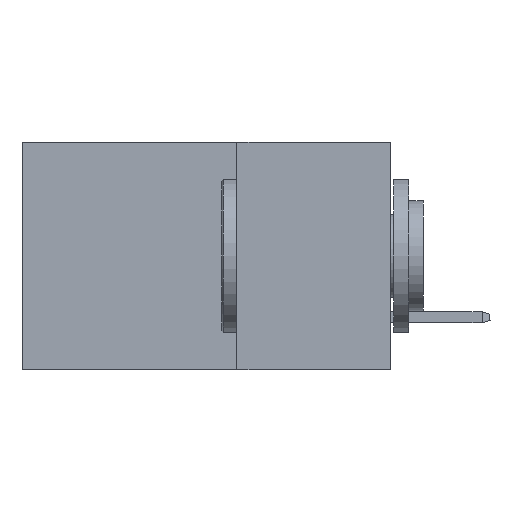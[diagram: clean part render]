
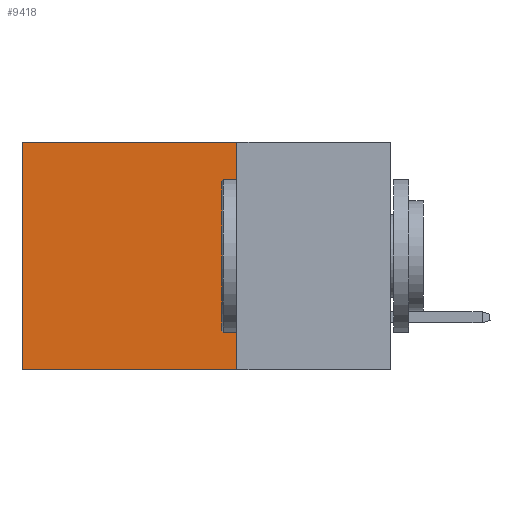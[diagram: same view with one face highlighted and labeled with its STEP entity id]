
A CAD part, left-side view. The second image highlights one B-rep face of the part: STEP entity #9418.
In plain terms, the highlighted planar face has unit normal (-1, 0, 0).
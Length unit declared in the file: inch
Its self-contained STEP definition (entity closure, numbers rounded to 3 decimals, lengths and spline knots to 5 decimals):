
#917 = VERTEX_POINT ( 'NONE', #14711 ) ;
#943 = LINE ( 'NONE', #15802, #15309 ) ;
#1311 = CARTESIAN_POINT ( 'NONE',  ( 0.2875, 0.6, -0.37 ) ) ;
#1991 = EDGE_CURVE ( 'NONE', #12289, #7194, #943, .T. ) ;
#3785 = CARTESIAN_POINT ( 'NONE',  ( 0.2875, 0.25, 0. ) ) ;
#4096 = ORIENTED_EDGE ( 'NONE', *, *, #1991, .T. ) ;
#4199 = LINE ( 'NONE', #7484, #7371 ) ;
#4247 = CARTESIAN_POINT ( 'NONE',  ( 0.2875, 0.25, 0. ) ) ;
#4553 = EDGE_CURVE ( 'NONE', #917, #7194, #4199, .T. ) ;
#4622 = CARTESIAN_POINT ( 'NONE',  ( 0.2875, 0.6, 0. ) ) ;
#6776 = FACE_OUTER_BOUND ( 'NONE', #11132, .T. ) ;
#7194 = VERTEX_POINT ( 'NONE', #1311 ) ;
#7371 = VECTOR ( 'NONE', #15582, 39.37008 ) ;
#7484 = CARTESIAN_POINT ( 'NONE',  ( 0.2875, 0.25, -0.37 ) ) ;
#7803 = PLANE ( 'NONE',  #10855 ) ;
#8778 = DIRECTION ( 'NONE',  ( 0., 0., -1. ) ) ;
#9418 = ADVANCED_FACE ( 'NONE', ( #6776 ), #7803, .F. ) ;
#9652 = EDGE_CURVE ( 'NONE', #16129, #12289, #13741, .T. ) ;
#10855 = AXIS2_PLACEMENT_3D ( 'NONE', #3785, #11821, #14344 ) ;
#11132 = EDGE_LOOP ( 'NONE', ( #4096, #11284, #17504, #13006 ) ) ;
#11284 = ORIENTED_EDGE ( 'NONE', *, *, #4553, .F. ) ;
#11478 = LINE ( 'NONE', #17088, #16330 ) ;
#11821 = DIRECTION ( 'NONE',  ( 1., 0., 0. ) ) ;
#12226 = DIRECTION ( 'NONE',  ( 0., 1., 0. ) ) ;
#12289 = VERTEX_POINT ( 'NONE', #4622 ) ;
#12922 = VECTOR ( 'NONE', #12226, 39.37008 ) ;
#13006 = ORIENTED_EDGE ( 'NONE', *, *, #9652, .T. ) ;
#13315 = CARTESIAN_POINT ( 'NONE',  ( 0.2875, 0.25, 0. ) ) ;
#13741 = LINE ( 'NONE', #4247, #12922 ) ;
#14344 = DIRECTION ( 'NONE',  ( 0., 0., -1. ) ) ;
#14573 = DIRECTION ( 'NONE',  ( 0., 0., -1. ) ) ;
#14711 = CARTESIAN_POINT ( 'NONE',  ( 0.2875, 0.25, -0.37 ) ) ;
#15309 = VECTOR ( 'NONE', #14573, 39.37008 ) ;
#15476 = EDGE_CURVE ( 'NONE', #16129, #917, #11478, .T. ) ;
#15582 = DIRECTION ( 'NONE',  ( 0., 1., 0. ) ) ;
#15802 = CARTESIAN_POINT ( 'NONE',  ( 0.2875, 0.6, 0. ) ) ;
#16129 = VERTEX_POINT ( 'NONE', #13315 ) ;
#16330 = VECTOR ( 'NONE', #8778, 39.37008 ) ;
#17088 = CARTESIAN_POINT ( 'NONE',  ( 0.2875, 0.25, 0. ) ) ;
#17504 = ORIENTED_EDGE ( 'NONE', *, *, #15476, .F. ) ;
